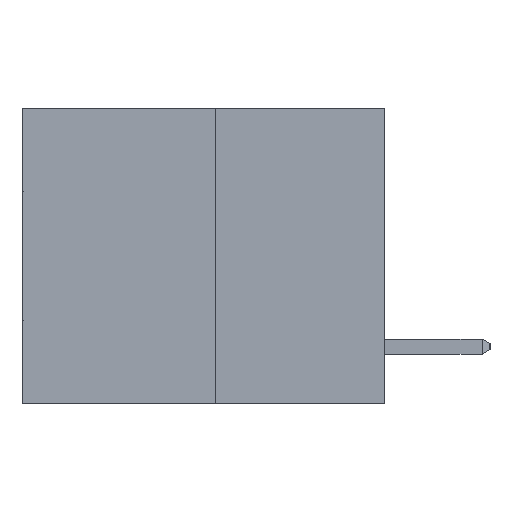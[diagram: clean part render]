
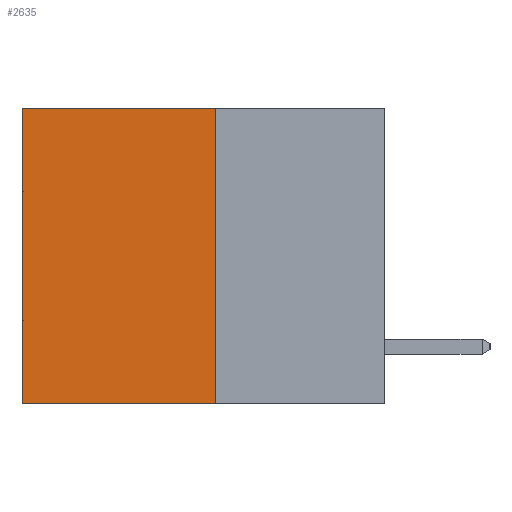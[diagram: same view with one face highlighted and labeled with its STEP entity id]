
A CAD part, left-side view. The second image highlights one B-rep face of the part: STEP entity #2635.
In plain terms, the highlighted planar face has unit normal (-1, 0, 0).
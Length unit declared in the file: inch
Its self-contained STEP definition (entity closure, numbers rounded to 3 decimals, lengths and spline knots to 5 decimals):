
#2635 = ADVANCED_FACE ( 'NONE', ( #14883 ), #20099, .F. ) ;
#3801 = EDGE_CURVE ( 'NONE', #21239, #7382, #19244, .T. ) ;
#5926 = VECTOR ( 'NONE', #17457, 39.37008 ) ;
#5955 = CARTESIAN_POINT ( 'NONE',  ( 0.3165, 0.28, -0.49 ) ) ;
#7382 = VERTEX_POINT ( 'NONE', #18183 ) ;
#8123 = LINE ( 'NONE', #15059, #18412 ) ;
#8274 = VECTOR ( 'NONE', #11993, 39.37008 ) ;
#8417 = LINE ( 'NONE', #23173, #18749 ) ;
#8453 = DIRECTION ( 'NONE',  ( 0., 0., -1. ) ) ;
#9027 = EDGE_CURVE ( 'NONE', #21239, #21691, #28933, .T. ) ;
#11993 = DIRECTION ( 'NONE',  ( 0., 1., 0. ) ) ;
#12523 = CARTESIAN_POINT ( 'NONE',  ( 0.3165, 0.6, -0.49 ) ) ;
#14883 = FACE_OUTER_BOUND ( 'NONE', #17819, .T. ) ;
#15059 = CARTESIAN_POINT ( 'NONE',  ( 0.3165, 0.6, -0.49 ) ) ;
#15520 = VERTEX_POINT ( 'NONE', #12523 ) ;
#16779 = CARTESIAN_POINT ( 'NONE',  ( 0.3165, 0.6, 0. ) ) ;
#17457 = DIRECTION ( 'NONE',  ( 0., 0., -1. ) ) ;
#17819 = EDGE_LOOP ( 'NONE', ( #18796, #24570, #28759, #24143 ) ) ;
#18183 = CARTESIAN_POINT ( 'NONE',  ( 0.3165, 0.28, -0.49 ) ) ;
#18412 = VECTOR ( 'NONE', #19602, 39.37008 ) ;
#18749 = VECTOR ( 'NONE', #20890, 39.37008 ) ;
#18796 = ORIENTED_EDGE ( 'NONE', *, *, #30439, .T. ) ;
#19244 = LINE ( 'NONE', #29189, #5926 ) ;
#19602 = DIRECTION ( 'NONE',  ( 0., 0., -1. ) ) ;
#20099 = PLANE ( 'NONE',  #26999 ) ;
#20890 = DIRECTION ( 'NONE',  ( 0., 1., 0. ) ) ;
#21239 = VERTEX_POINT ( 'NONE', #24336 ) ;
#21395 = CARTESIAN_POINT ( 'NONE',  ( 0.3165, 0.28, 0. ) ) ;
#21691 = VERTEX_POINT ( 'NONE', #16779 ) ;
#22467 = DIRECTION ( 'NONE',  ( 1., 0., 0. ) ) ;
#23173 = CARTESIAN_POINT ( 'NONE',  ( 0.3165, 0.28, -0.49 ) ) ;
#24143 = ORIENTED_EDGE ( 'NONE', *, *, #9027, .T. ) ;
#24336 = CARTESIAN_POINT ( 'NONE',  ( 0.3165, 0.28, 0. ) ) ;
#24570 = ORIENTED_EDGE ( 'NONE', *, *, #24614, .F. ) ;
#24614 = EDGE_CURVE ( 'NONE', #7382, #15520, #8417, .T. ) ;
#26999 = AXIS2_PLACEMENT_3D ( 'NONE', #5955, #22467, #8453 ) ;
#28759 = ORIENTED_EDGE ( 'NONE', *, *, #3801, .F. ) ;
#28933 = LINE ( 'NONE', #21395, #8274 ) ;
#29189 = CARTESIAN_POINT ( 'NONE',  ( 0.3165, 0.28, -0.49 ) ) ;
#30439 = EDGE_CURVE ( 'NONE', #21691, #15520, #8123, .T. ) ;
